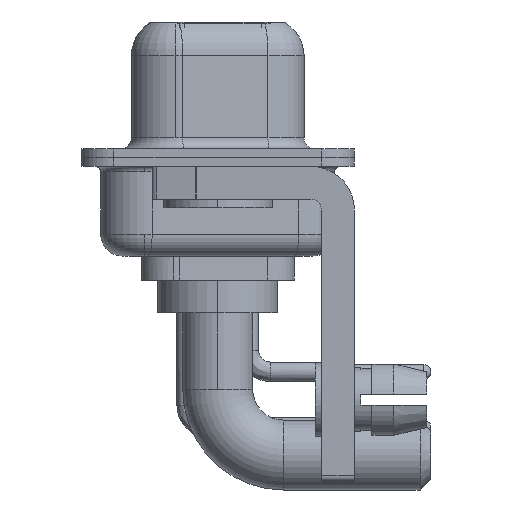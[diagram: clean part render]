
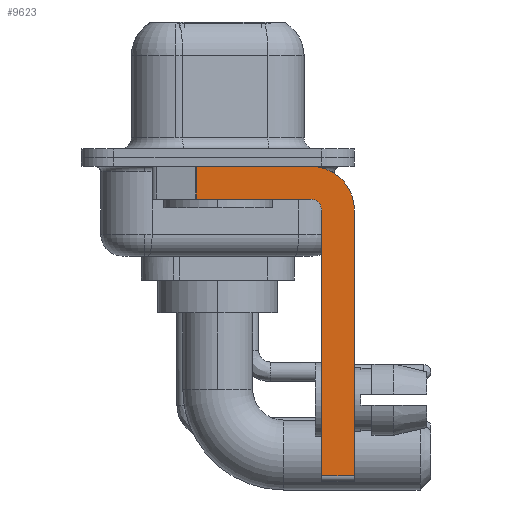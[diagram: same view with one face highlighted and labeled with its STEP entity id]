
A CAD part, left-side view. The second image highlights one B-rep face of the part: STEP entity #9623.
In plain terms, the highlighted planar face has unit normal (-1, 0, 0).
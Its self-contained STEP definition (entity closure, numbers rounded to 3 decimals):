
#155 = CARTESIAN_POINT ( 'NONE',  ( -2.9, -4.25, -2.4 ) ) ;
#217 = PLANE ( 'NONE',  #11849 ) ;
#332 = CIRCLE ( 'NONE', #14111, 2. ) ;
#346 = FACE_OUTER_BOUND ( 'NONE', #8654, .T. ) ;
#474 = ORIENTED_EDGE ( 'NONE', *, *, #17892, .F. ) ;
#553 = DIRECTION ( 'NONE',  ( 0., -1., 0. ) ) ;
#2017 = CARTESIAN_POINT ( 'NONE',  ( -2.9, -4.75, -14.8 ) ) ;
#2040 = DIRECTION ( 'NONE',  ( 0., 1., 0. ) ) ;
#2072 = DIRECTION ( 'NONE',  ( 0., 0., -1. ) ) ;
#2184 = ORIENTED_EDGE ( 'NONE', *, *, #4926, .F. ) ;
#2319 = VERTEX_POINT ( 'NONE', #9098 ) ;
#2344 = CARTESIAN_POINT ( 'NONE',  ( -2.9, 0.978, -0.4 ) ) ;
#3434 = VECTOR ( 'NONE', #14053, 1000. ) ;
#3998 = CARTESIAN_POINT ( 'NONE',  ( -2.9, -4.25, -1.9 ) ) ;
#4294 = EDGE_CURVE ( 'NONE', #11347, #21012, #9797, .T. ) ;
#4442 = LINE ( 'NONE', #16034, #3434 ) ;
#4642 = ORIENTED_EDGE ( 'NONE', *, *, #17034, .T. ) ;
#4746 = VECTOR ( 'NONE', #21138, 1000. ) ;
#4926 = EDGE_CURVE ( 'NONE', #18986, #2319, #332, .T. ) ;
#5383 = ORIENTED_EDGE ( 'NONE', *, *, #11289, .T. ) ;
#5888 = VERTEX_POINT ( 'NONE', #15236 ) ;
#5933 = LINE ( 'NONE', #13583, #11767 ) ;
#5947 = LINE ( 'NONE', #2017, #4746 ) ;
#6960 = EDGE_CURVE ( 'NONE', #16672, #11347, #13302, .T. ) ;
#7429 = EDGE_CURVE ( 'NONE', #2319, #5888, #5933, .T. ) ;
#7852 = CARTESIAN_POINT ( 'NONE',  ( -2.9, -4.25, -2.4 ) ) ;
#8010 = CARTESIAN_POINT ( 'NONE',  ( -2.9, -4.25, -2.4 ) ) ;
#8148 = DIRECTION ( 'NONE',  ( 0., 0., -1. ) ) ;
#8375 = DIRECTION ( 'NONE',  ( -1., 0., 0. ) ) ;
#8654 = EDGE_LOOP ( 'NONE', ( #474, #5383, #10590, #23167, #18834, #4642, #15174, #2184 ) ) ;
#8684 = VERTEX_POINT ( 'NONE', #16463 ) ;
#9098 = CARTESIAN_POINT ( 'NONE',  ( -2.9, -6.25, -2.4 ) ) ;
#9560 = CARTESIAN_POINT ( 'NONE',  ( -2.9, -4.25, -0.4 ) ) ;
#9623 = ADVANCED_FACE ( 'NONE', ( #346 ), #217, .F. ) ;
#9706 = DIRECTION ( 'NONE',  ( 1., 0., 0. ) ) ;
#9797 = LINE ( 'NONE', #3998, #12417 ) ;
#10538 = EDGE_CURVE ( 'NONE', #8684, #16672, #5947, .T. ) ;
#10572 = AXIS2_PLACEMENT_3D ( 'NONE', #8010, #8375, #15913 ) ;
#10590 = ORIENTED_EDGE ( 'NONE', *, *, #4294, .F. ) ;
#11289 = EDGE_CURVE ( 'NONE', #20565, #21012, #22286, .T. ) ;
#11347 = VERTEX_POINT ( 'NONE', #24142 ) ;
#11767 = VECTOR ( 'NONE', #8148, 1000. ) ;
#11849 = AXIS2_PLACEMENT_3D ( 'NONE', #7852, #9706, #2072 ) ;
#12417 = VECTOR ( 'NONE', #2040, 1000. ) ;
#13026 = VECTOR ( 'NONE', #553, 1000. ) ;
#13047 = VECTOR ( 'NONE', #22411, 1000. ) ;
#13230 = DIRECTION ( 'NONE',  ( 1., 0., 0. ) ) ;
#13302 = CIRCLE ( 'NONE', #10572, 0.5 ) ;
#13583 = CARTESIAN_POINT ( 'NONE',  ( -2.9, -6.25, -2.4 ) ) ;
#14053 = DIRECTION ( 'NONE',  ( 0., -1., 0. ) ) ;
#14111 = AXIS2_PLACEMENT_3D ( 'NONE', #155, #13230, #20895 ) ;
#15174 = ORIENTED_EDGE ( 'NONE', *, *, #7429, .F. ) ;
#15236 = CARTESIAN_POINT ( 'NONE',  ( -2.9, -6.25, -14.55 ) ) ;
#15913 = DIRECTION ( 'NONE',  ( 0., 0., 1. ) ) ;
#15972 = CARTESIAN_POINT ( 'NONE',  ( -2.9, 3., -0.4 ) ) ;
#16034 = CARTESIAN_POINT ( 'NONE',  ( -2.9, -4.25, -14.55 ) ) ;
#16463 = CARTESIAN_POINT ( 'NONE',  ( -2.9, -4.75, -14.55 ) ) ;
#16474 = CARTESIAN_POINT ( 'NONE',  ( -2.9, 0.978, -1.9 ) ) ;
#16672 = VERTEX_POINT ( 'NONE', #21985 ) ;
#17034 = EDGE_CURVE ( 'NONE', #8684, #5888, #4442, .T. ) ;
#17584 = LINE ( 'NONE', #15972, #13026 ) ;
#17852 = CARTESIAN_POINT ( 'NONE',  ( -2.9, 0.978, -1.9 ) ) ;
#17892 = EDGE_CURVE ( 'NONE', #20565, #18986, #17584, .T. ) ;
#18834 = ORIENTED_EDGE ( 'NONE', *, *, #10538, .F. ) ;
#18986 = VERTEX_POINT ( 'NONE', #9560 ) ;
#20565 = VERTEX_POINT ( 'NONE', #2344 ) ;
#20895 = DIRECTION ( 'NONE',  ( 0., 0., -1. ) ) ;
#21012 = VERTEX_POINT ( 'NONE', #17852 ) ;
#21138 = DIRECTION ( 'NONE',  ( 0., 0., 1. ) ) ;
#21985 = CARTESIAN_POINT ( 'NONE',  ( -2.9, -4.75, -2.4 ) ) ;
#22286 = LINE ( 'NONE', #16474, #13047 ) ;
#22411 = DIRECTION ( 'NONE',  ( 0., 0., -1. ) ) ;
#23167 = ORIENTED_EDGE ( 'NONE', *, *, #6960, .F. ) ;
#24142 = CARTESIAN_POINT ( 'NONE',  ( -2.9, -4.25, -1.9 ) ) ;
